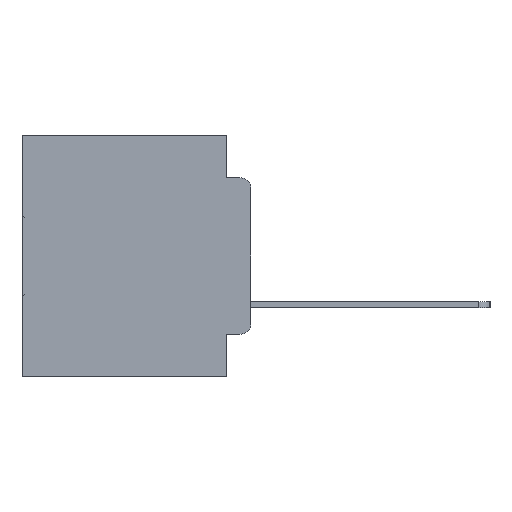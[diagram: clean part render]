
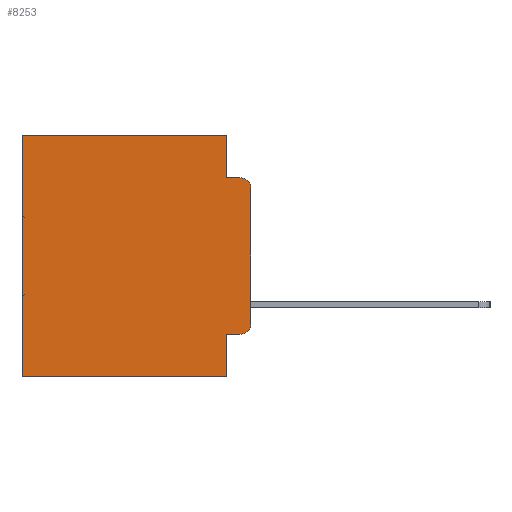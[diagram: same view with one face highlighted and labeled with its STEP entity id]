
A CAD part, left-side view. The second image highlights one B-rep face of the part: STEP entity #8253.
In plain terms, the highlighted planar face has unit normal (-1, 0, 0).
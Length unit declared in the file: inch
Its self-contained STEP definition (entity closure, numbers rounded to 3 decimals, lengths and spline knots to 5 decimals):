
#204 = DIRECTION ( 'NONE',  ( 0., 0., -1. ) ) ;
#1353 = CARTESIAN_POINT ( 'NONE',  ( 0.298, 0.051, -0.0885 ) ) ;
#1849 = EDGE_CURVE ( 'NONE', #10259, #24029, #32732, .T. ) ;
#1965 = CARTESIAN_POINT ( 'NONE',  ( 0.298, 0.051, -0.5 ) ) ;
#1976 = VERTEX_POINT ( 'NONE', #19704 ) ;
#2304 = CIRCLE ( 'NONE', #18029, 0.02 ) ;
#2728 = LINE ( 'NONE', #10486, #16580 ) ;
#2740 = EDGE_CURVE ( 'NONE', #10174, #12638, #17977, .T. ) ;
#3155 = CARTESIAN_POINT ( 'NONE',  ( 0.298, 0., 0. ) ) ;
#3791 = VERTEX_POINT ( 'NONE', #10913 ) ;
#3793 = DIRECTION ( 'NONE',  ( -1., 0., 0. ) ) ;
#4950 = EDGE_LOOP ( 'NONE', ( #34727, #18992, #32822, #20635, #7865, #18588, #21076, #9193, #19858, #23707 ) ) ;
#5620 = VECTOR ( 'NONE', #20723, 39.37008 ) ;
#5995 = DIRECTION ( 'NONE',  ( 0., 0., -1. ) ) ;
#6202 = CARTESIAN_POINT ( 'NONE',  ( 0.298, 0.051, 0. ) ) ;
#6769 = CARTESIAN_POINT ( 'NONE',  ( 0.298, 0.02, -0.1085 ) ) ;
#7865 = ORIENTED_EDGE ( 'NONE', *, *, #1849, .T. ) ;
#8253 = ADVANCED_FACE ( 'NONE', ( #9641 ), #32577, .F. ) ;
#8918 = CARTESIAN_POINT ( 'NONE',  ( 0.298, 0.02, -0.4115 ) ) ;
#9193 = ORIENTED_EDGE ( 'NONE', *, *, #22246, .F. ) ;
#9505 = VECTOR ( 'NONE', #19077, 39.37008 ) ;
#9548 = DIRECTION ( 'NONE',  ( 0., 0., -1. ) ) ;
#9641 = FACE_OUTER_BOUND ( 'NONE', #4950, .T. ) ;
#10174 = VERTEX_POINT ( 'NONE', #8918 ) ;
#10259 = VERTEX_POINT ( 'NONE', #14816 ) ;
#10486 = CARTESIAN_POINT ( 'NONE',  ( 0.298, 0.473, 0. ) ) ;
#10913 = CARTESIAN_POINT ( 'NONE',  ( 0.298, 0.473, -0.5 ) ) ;
#11393 = VERTEX_POINT ( 'NONE', #29744 ) ;
#11529 = AXIS2_PLACEMENT_3D ( 'NONE', #3155, #22301, #5995 ) ;
#11814 = CARTESIAN_POINT ( 'NONE',  ( 0.298, 0.473, 0. ) ) ;
#11862 = VERTEX_POINT ( 'NONE', #1965 ) ;
#12638 = VERTEX_POINT ( 'NONE', #13625 ) ;
#13379 = LINE ( 'NONE', #29054, #26715 ) ;
#13625 = CARTESIAN_POINT ( 'NONE',  ( 0.298, 0., -0.3915 ) ) ;
#13862 = LINE ( 'NONE', #1353, #5620 ) ;
#14232 = CARTESIAN_POINT ( 'NONE',  ( 0.298, 0.02, -0.0885 ) ) ;
#14656 = AXIS2_PLACEMENT_3D ( 'NONE', #20250, #3793, #22911 ) ;
#14816 = CARTESIAN_POINT ( 'NONE',  ( 0.298, 0.051, 0. ) ) ;
#15637 = CARTESIAN_POINT ( 'NONE',  ( 0.298, 0., -0.5 ) ) ;
#15934 = DIRECTION ( 'NONE',  ( 0., 0., -1. ) ) ;
#16062 = LINE ( 'NONE', #15637, #28425 ) ;
#16398 = CARTESIAN_POINT ( 'NONE',  ( 0.298, 0.051, -0.4115 ) ) ;
#16580 = VECTOR ( 'NONE', #31711, 39.37008 ) ;
#17433 = VECTOR ( 'NONE', #204, 39.37008 ) ;
#17977 = CIRCLE ( 'NONE', #14656, 0.02 ) ;
#18029 = AXIS2_PLACEMENT_3D ( 'NONE', #6769, #25673, #9548 ) ;
#18481 = EDGE_CURVE ( 'NONE', #24674, #34788, #13862, .T. ) ;
#18588 = ORIENTED_EDGE ( 'NONE', *, *, #21571, .T. ) ;
#18903 = VECTOR ( 'NONE', #24004, 39.37008 ) ;
#18992 = ORIENTED_EDGE ( 'NONE', *, *, #21369, .T. ) ;
#19077 = DIRECTION ( 'NONE',  ( 0., -1., 0. ) ) ;
#19704 = CARTESIAN_POINT ( 'NONE',  ( 0.298, 0., -0.1085 ) ) ;
#19782 = LINE ( 'NONE', #6202, #30375 ) ;
#19858 = ORIENTED_EDGE ( 'NONE', *, *, #31563, .T. ) ;
#19939 = CARTESIAN_POINT ( 'NONE',  ( 0.298, 0.051, -0.0885 ) ) ;
#20250 = CARTESIAN_POINT ( 'NONE',  ( 0.298, 0.02, -0.3915 ) ) ;
#20635 = ORIENTED_EDGE ( 'NONE', *, *, #30292, .F. ) ;
#20723 = DIRECTION ( 'NONE',  ( 0., -1., 0. ) ) ;
#21076 = ORIENTED_EDGE ( 'NONE', *, *, #23821, .F. ) ;
#21369 = EDGE_CURVE ( 'NONE', #1976, #34788, #2304, .T. ) ;
#21571 = EDGE_CURVE ( 'NONE', #24029, #3791, #2728, .T. ) ;
#22246 = EDGE_CURVE ( 'NONE', #11393, #11862, #30887, .T. ) ;
#22301 = DIRECTION ( 'NONE',  ( 1., 0., 0. ) ) ;
#22911 = DIRECTION ( 'NONE',  ( 0., 0., -1. ) ) ;
#23707 = ORIENTED_EDGE ( 'NONE', *, *, #2740, .T. ) ;
#23821 = EDGE_CURVE ( 'NONE', #11862, #3791, #16062, .T. ) ;
#24004 = DIRECTION ( 'NONE',  ( 0., 1., 0. ) ) ;
#24029 = VERTEX_POINT ( 'NONE', #11814 ) ;
#24674 = VERTEX_POINT ( 'NONE', #19939 ) ;
#24853 = CARTESIAN_POINT ( 'NONE',  ( 0.298, 0.051, 0. ) ) ;
#25261 = DIRECTION ( 'NONE',  ( 0., 0., -1. ) ) ;
#25673 = DIRECTION ( 'NONE',  ( -1., 0., 0. ) ) ;
#26617 = CARTESIAN_POINT ( 'NONE',  ( 0.298, 0., 0. ) ) ;
#26715 = VECTOR ( 'NONE', #15934, 39.37008 ) ;
#28425 = VECTOR ( 'NONE', #28891, 39.37008 ) ;
#28814 = EDGE_CURVE ( 'NONE', #1976, #12638, #13379, .T. ) ;
#28891 = DIRECTION ( 'NONE',  ( 0., 1., 0. ) ) ;
#29054 = CARTESIAN_POINT ( 'NONE',  ( 0.298, 0., 0. ) ) ;
#29744 = CARTESIAN_POINT ( 'NONE',  ( 0.298, 0.051, -0.4115 ) ) ;
#30292 = EDGE_CURVE ( 'NONE', #10259, #24674, #19782, .T. ) ;
#30375 = VECTOR ( 'NONE', #25261, 39.37008 ) ;
#30736 = LINE ( 'NONE', #16398, #9505 ) ;
#30887 = LINE ( 'NONE', #24853, #17433 ) ;
#31563 = EDGE_CURVE ( 'NONE', #11393, #10174, #30736, .T. ) ;
#31711 = DIRECTION ( 'NONE',  ( 0., 0., -1. ) ) ;
#32577 = PLANE ( 'NONE',  #11529 ) ;
#32732 = LINE ( 'NONE', #26617, #18903 ) ;
#32822 = ORIENTED_EDGE ( 'NONE', *, *, #18481, .F. ) ;
#34727 = ORIENTED_EDGE ( 'NONE', *, *, #28814, .F. ) ;
#34788 = VERTEX_POINT ( 'NONE', #14232 ) ;
